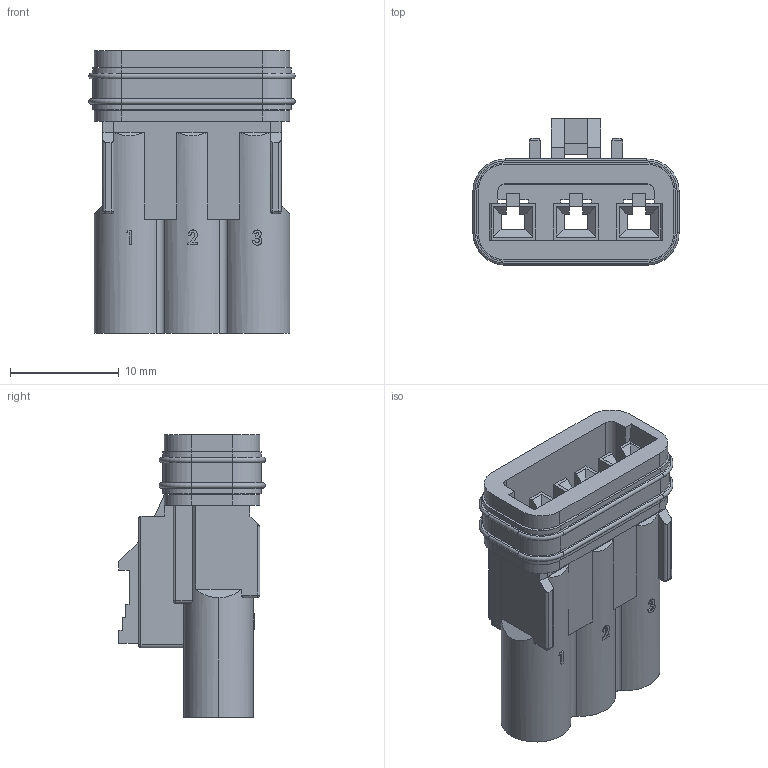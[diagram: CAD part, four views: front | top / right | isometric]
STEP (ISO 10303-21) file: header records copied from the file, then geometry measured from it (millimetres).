
FILE_DESCRIPTION (( 'STEP AP214' ), '1' );
FILE_NAME ('570-003-000-200.STEP', '2020-07-30T14:46:26', ( '' ), ( '' ), 'SwSTEP 2.0', 'SolidWorks 2020', '' );
FILE_SCHEMA (( 'AUTOMOTIVE_DESIGN' ));
Length unit declared in the file: millimetre
Products named in the file (3): 570-003-000-200_Rubber; 570-003-000-200_Housing; 570-003-000-200
Assembly tree (2 placements, depth 2):
  570-003-000-200
    570-003-000-200_Housing
    570-003-000-200_Rubber
Bounding box: 18.98 x 13.49 x 26 mm (x, y, z)
Volume: 1796.6 mm3; surface area: 3997.4 mm2
Topology: 2 solids, 2 shells, 425 faces, 1174 edges, 752 vertices
Faces by surface type: plane 272, cylinder 100, torus 24, bspline 19, sphere 10
Entity records: 14379 total; most frequent: CARTESIAN_POINT 3527, ORIENTED_EDGE 2328, DIRECTION 2159, EDGE_CURVE 1164, VECTOR 813, LINE 813, VERTEX_POINT 752, AXIS2_PLACEMENT_3D 673
